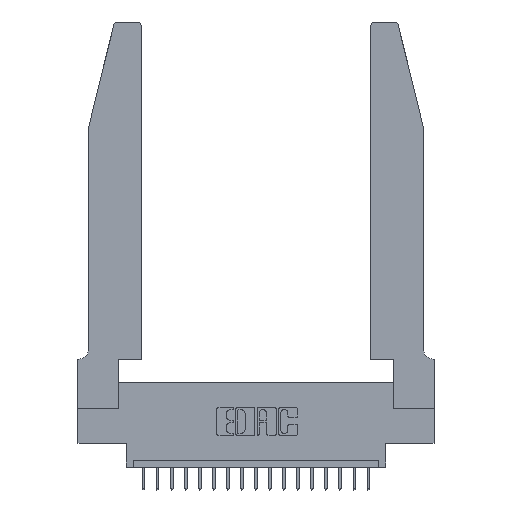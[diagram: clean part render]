
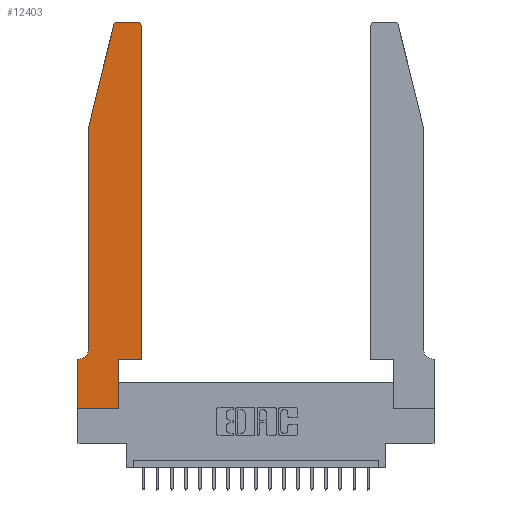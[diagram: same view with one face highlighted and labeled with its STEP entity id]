
A CAD part, top view. The second image highlights one B-rep face of the part: STEP entity #12403.
In plain terms, the highlighted planar face has unit normal (0, 0, 1).
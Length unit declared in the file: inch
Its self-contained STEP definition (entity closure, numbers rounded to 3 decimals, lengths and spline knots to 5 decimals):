
#260 = DIRECTION ( 'NONE',  ( -1., 0., 0. ) ) ;
#605 = DIRECTION ( 'NONE',  ( 0., -1., 0. ) ) ;
#655 = ORIENTED_EDGE ( 'NONE', *, *, #3784, .T. ) ;
#659 = VERTEX_POINT ( 'NONE', #12028 ) ;
#837 = EDGE_CURVE ( 'NONE', #7233, #14519, #1740, .T. ) ;
#929 = VERTEX_POINT ( 'NONE', #10452 ) ;
#1440 = VECTOR ( 'NONE', #13974, 39.37008 ) ;
#1453 = VECTOR ( 'NONE', #18388, 39.37008 ) ;
#1620 = DIRECTION ( 'NONE',  ( 0., -1., 0. ) ) ;
#1687 = VECTOR ( 'NONE', #9047, 39.37008 ) ;
#1718 = VERTEX_POINT ( 'NONE', #5511 ) ;
#1740 = LINE ( 'NONE', #16333, #13755 ) ;
#2095 = VERTEX_POINT ( 'NONE', #3096 ) ;
#2228 = CARTESIAN_POINT ( 'NONE',  ( 0., 0., 0.37 ) ) ;
#2472 = EDGE_CURVE ( 'NONE', #2095, #929, #4494, .T. ) ;
#2519 = CARTESIAN_POINT ( 'NONE',  ( 0.284, 2.72, 0.37 ) ) ;
#2838 = CARTESIAN_POINT ( 'NONE',  ( 0.0755, 0.35, 0.37 ) ) ;
#3096 = CARTESIAN_POINT ( 'NONE',  ( 0., 0., 0.37 ) ) ;
#3144 = LINE ( 'NONE', #11817, #15211 ) ;
#3267 = FACE_OUTER_BOUND ( 'NONE', #8099, .T. ) ;
#3273 = VERTEX_POINT ( 'NONE', #14719 ) ;
#3784 = EDGE_CURVE ( 'NONE', #929, #7233, #14443, .T. ) ;
#3816 = DIRECTION ( 'NONE',  ( 1., 0., 0. ) ) ;
#3888 = DIRECTION ( 'NONE',  ( 0., 0., 1. ) ) ;
#3894 = VERTEX_POINT ( 'NONE', #9119 ) ;
#4044 = CARTESIAN_POINT ( 'NONE',  ( 0.4505, 0.35, 0.37 ) ) ;
#4064 = CARTESIAN_POINT ( 'NONE',  ( 0.4505, 0.35, 0.37 ) ) ;
#4144 = CIRCLE ( 'NONE', #11445, 0.07 ) ;
#4150 = DIRECTION ( 'NONE',  ( 1., 0., 0. ) ) ;
#4208 = CARTESIAN_POINT ( 'NONE',  ( 0.25487, 2.72718, 0.37 ) ) ;
#4494 = LINE ( 'NONE', #2228, #1453 ) ;
#4694 = AXIS2_PLACEMENT_3D ( 'NONE', #17539, #14331, #14402 ) ;
#4931 = VECTOR ( 'NONE', #10802, 39.37008 ) ;
#5434 = AXIS2_PLACEMENT_3D ( 'NONE', #2519, #13958, #4150 ) ;
#5467 = EDGE_CURVE ( 'NONE', #20332, #20710, #10305, .T. ) ;
#5511 = CARTESIAN_POINT ( 'NONE',  ( 0.4505, 2.72, 0.37 ) ) ;
#5640 = ORIENTED_EDGE ( 'NONE', *, *, #8846, .T. ) ;
#5916 = VERTEX_POINT ( 'NONE', #13803 ) ;
#7203 = DIRECTION ( 'NONE',  ( -1., 0., 0. ) ) ;
#7233 = VERTEX_POINT ( 'NONE', #10800 ) ;
#7740 = EDGE_CURVE ( 'NONE', #3894, #2095, #17595, .T. ) ;
#8099 = EDGE_LOOP ( 'NONE', ( #5640, #20431, #18069, #16408, #17431, #17698, #17547, #19103, #655, #15280, #15252, #10609 ) ) ;
#8252 = CARTESIAN_POINT ( 'NONE',  ( 0.0755, 2., 0.37 ) ) ;
#8260 = LINE ( 'NONE', #15256, #4931 ) ;
#8846 = EDGE_CURVE ( 'NONE', #3273, #20332, #3144, .T. ) ;
#9047 = DIRECTION ( 'NONE',  ( 0., 1., 0. ) ) ;
#9119 = CARTESIAN_POINT ( 'NONE',  ( 0., 0.35, 0.37 ) ) ;
#9277 = EDGE_CURVE ( 'NONE', #20710, #16420, #8260, .T. ) ;
#9773 = LINE ( 'NONE', #8252, #11043 ) ;
#10305 = CIRCLE ( 'NONE', #5434, 0.03 ) ;
#10405 = CARTESIAN_POINT ( 'NONE',  ( 0.2865, 0.35, 0.37 ) ) ;
#10429 = EDGE_CURVE ( 'NONE', #1718, #3273, #19675, .T. ) ;
#10452 = CARTESIAN_POINT ( 'NONE',  ( 0.2865, 0., 0.37 ) ) ;
#10609 = ORIENTED_EDGE ( 'NONE', *, *, #10429, .T. ) ;
#10800 = CARTESIAN_POINT ( 'NONE',  ( 0.2865, 0.35, 0.37 ) ) ;
#10802 = DIRECTION ( 'NONE',  ( -0.239, -0.971, 0. ) ) ;
#10900 = CARTESIAN_POINT ( 'NONE',  ( 0., 0., 0.37 ) ) ;
#11043 = VECTOR ( 'NONE', #1620, 39.37008 ) ;
#11445 = AXIS2_PLACEMENT_3D ( 'NONE', #14976, #13381, #260 ) ;
#11817 = CARTESIAN_POINT ( 'NONE',  ( 0.2605, 2.75, 0.37 ) ) ;
#12028 = CARTESIAN_POINT ( 'NONE',  ( 0.0755, 0.42, 0.37 ) ) ;
#12403 = ADVANCED_FACE ( 'NONE', ( #3267 ), #12663, .T. ) ;
#12663 = PLANE ( 'NONE',  #4694 ) ;
#13381 = DIRECTION ( 'NONE',  ( 0., 0., -1. ) ) ;
#13447 = CARTESIAN_POINT ( 'NONE',  ( 0.284, 2.75, 0.37 ) ) ;
#13755 = VECTOR ( 'NONE', #17966, 39.37008 ) ;
#13803 = CARTESIAN_POINT ( 'NONE',  ( 0.0055, 0.35, 0.37 ) ) ;
#13825 = CARTESIAN_POINT ( 'NONE',  ( 0.4205, 2.72, 0.37 ) ) ;
#13958 = DIRECTION ( 'NONE',  ( 0., 0., 1. ) ) ;
#13974 = DIRECTION ( 'NONE',  ( 0., 1., 0. ) ) ;
#14331 = DIRECTION ( 'NONE',  ( 0., 0., 1. ) ) ;
#14402 = DIRECTION ( 'NONE',  ( 1., 0., 0. ) ) ;
#14443 = LINE ( 'NONE', #10405, #1440 ) ;
#14519 = VERTEX_POINT ( 'NONE', #4064 ) ;
#14719 = CARTESIAN_POINT ( 'NONE',  ( 0.4205, 2.75, 0.37 ) ) ;
#14976 = CARTESIAN_POINT ( 'NONE',  ( 0.0055, 0.42, 0.37 ) ) ;
#15211 = VECTOR ( 'NONE', #7203, 39.37008 ) ;
#15252 = ORIENTED_EDGE ( 'NONE', *, *, #21137, .T. ) ;
#15256 = CARTESIAN_POINT ( 'NONE',  ( 0.0755, 2., 0.37 ) ) ;
#15280 = ORIENTED_EDGE ( 'NONE', *, *, #837, .T. ) ;
#15289 = CARTESIAN_POINT ( 'NONE',  ( 0.0755, 2., 0.37 ) ) ;
#15753 = LINE ( 'NONE', #4044, #1687 ) ;
#16162 = DIRECTION ( 'NONE',  ( -1., 0., 0. ) ) ;
#16301 = EDGE_CURVE ( 'NONE', #5916, #3894, #16970, .T. ) ;
#16333 = CARTESIAN_POINT ( 'NONE',  ( 0.4505, 0.35, 0.37 ) ) ;
#16408 = ORIENTED_EDGE ( 'NONE', *, *, #16718, .T. ) ;
#16420 = VERTEX_POINT ( 'NONE', #15289 ) ;
#16718 = EDGE_CURVE ( 'NONE', #16420, #659, #9773, .T. ) ;
#16825 = EDGE_CURVE ( 'NONE', #659, #5916, #4144, .T. ) ;
#16970 = LINE ( 'NONE', #2838, #19225 ) ;
#17431 = ORIENTED_EDGE ( 'NONE', *, *, #16825, .T. ) ;
#17539 = CARTESIAN_POINT ( 'NONE',  ( 0., 0.35, 0.37 ) ) ;
#17547 = ORIENTED_EDGE ( 'NONE', *, *, #7740, .T. ) ;
#17595 = LINE ( 'NONE', #10900, #17865 ) ;
#17698 = ORIENTED_EDGE ( 'NONE', *, *, #16301, .T. ) ;
#17865 = VECTOR ( 'NONE', #605, 39.37008 ) ;
#17966 = DIRECTION ( 'NONE',  ( 1., 0., 0. ) ) ;
#18069 = ORIENTED_EDGE ( 'NONE', *, *, #9277, .T. ) ;
#18388 = DIRECTION ( 'NONE',  ( 1., 0., 0. ) ) ;
#19103 = ORIENTED_EDGE ( 'NONE', *, *, #2472, .T. ) ;
#19225 = VECTOR ( 'NONE', #16162, 39.37008 ) ;
#19675 = CIRCLE ( 'NONE', #20611, 0.03 ) ;
#20332 = VERTEX_POINT ( 'NONE', #13447 ) ;
#20431 = ORIENTED_EDGE ( 'NONE', *, *, #5467, .T. ) ;
#20611 = AXIS2_PLACEMENT_3D ( 'NONE', #13825, #3888, #3816 ) ;
#20710 = VERTEX_POINT ( 'NONE', #4208 ) ;
#21137 = EDGE_CURVE ( 'NONE', #14519, #1718, #15753, .T. ) ;
